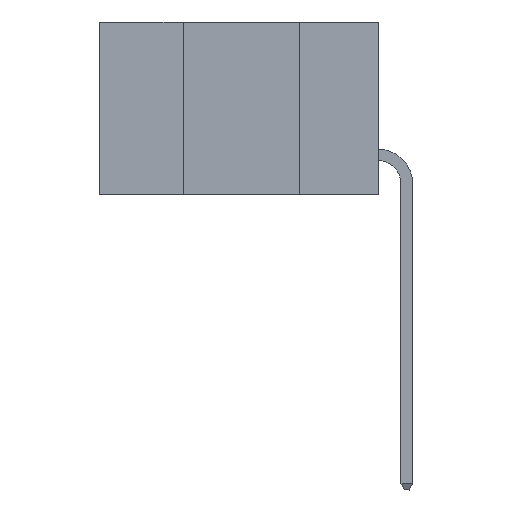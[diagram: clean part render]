
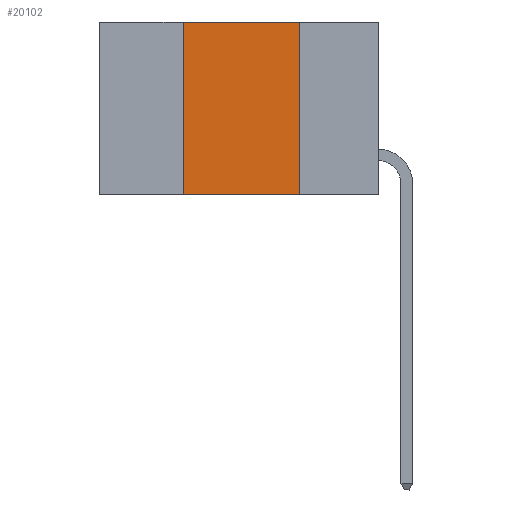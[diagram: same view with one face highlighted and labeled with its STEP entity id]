
A CAD part, left-side view. The second image highlights one B-rep face of the part: STEP entity #20102.
In plain terms, the highlighted planar face has unit normal (-1, 0, 0).
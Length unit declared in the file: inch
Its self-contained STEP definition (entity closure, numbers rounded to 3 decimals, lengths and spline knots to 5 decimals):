
#1355 = VECTOR ( 'NONE', #16091, 39.37008 ) ;
#1516 = EDGE_CURVE ( 'NONE', #18307, #8647, #14158, .T. ) ;
#3431 = PLANE ( 'NONE',  #28466 ) ;
#4315 = CARTESIAN_POINT ( 'NONE',  ( 0., 0.42, 0. ) ) ;
#7027 = LINE ( 'NONE', #16688, #25282 ) ;
#8188 = LINE ( 'NONE', #4315, #19424 ) ;
#8274 = DIRECTION ( 'NONE',  ( 1., 0., 0. ) ) ;
#8341 = CARTESIAN_POINT ( 'NONE',  ( 0., 0.17, 0. ) ) ;
#8647 = VERTEX_POINT ( 'NONE', #8341 ) ;
#9548 = DIRECTION ( 'NONE',  ( 0., -1., 0. ) ) ;
#10759 = ORIENTED_EDGE ( 'NONE', *, *, #26162, .F. ) ;
#11028 = VERTEX_POINT ( 'NONE', #11804 ) ;
#11540 = ORIENTED_EDGE ( 'NONE', *, *, #26784, .F. ) ;
#11804 = CARTESIAN_POINT ( 'NONE',  ( 0., 0.17, -0.37 ) ) ;
#13955 = EDGE_LOOP ( 'NONE', ( #10759, #23388, #11540, #28905 ) ) ;
#14158 = LINE ( 'NONE', #28954, #1355 ) ;
#16091 = DIRECTION ( 'NONE',  ( 0., -1., 0. ) ) ;
#16284 = VERTEX_POINT ( 'NONE', #22019 ) ;
#16291 = DIRECTION ( 'NONE',  ( 0., 0., 1. ) ) ;
#16688 = CARTESIAN_POINT ( 'NONE',  ( 0., 0.6, -0.37 ) ) ;
#18307 = VERTEX_POINT ( 'NONE', #29461 ) ;
#18661 = FACE_OUTER_BOUND ( 'NONE', #13955, .T. ) ;
#18730 = CARTESIAN_POINT ( 'NONE',  ( 0., 0.17, 0. ) ) ;
#19424 = VECTOR ( 'NONE', #16291, 39.37008 ) ;
#20102 = ADVANCED_FACE ( 'NONE', ( #18661 ), #3431, .F. ) ;
#22019 = CARTESIAN_POINT ( 'NONE',  ( 0., 0.42, -0.37 ) ) ;
#23388 = ORIENTED_EDGE ( 'NONE', *, *, #1516, .F. ) ;
#24928 = DIRECTION ( 'NONE',  ( 0., 0., -1. ) ) ;
#25282 = VECTOR ( 'NONE', #9548, 39.37008 ) ;
#25345 = VECTOR ( 'NONE', #28113, 39.37008 ) ;
#26162 = EDGE_CURVE ( 'NONE', #8647, #11028, #26773, .T. ) ;
#26773 = LINE ( 'NONE', #18730, #25345 ) ;
#26784 = EDGE_CURVE ( 'NONE', #16284, #18307, #8188, .T. ) ;
#27134 = CARTESIAN_POINT ( 'NONE',  ( 0., 0.6, 0. ) ) ;
#28113 = DIRECTION ( 'NONE',  ( 0., 0., -1. ) ) ;
#28466 = AXIS2_PLACEMENT_3D ( 'NONE', #27134, #8274, #24928 ) ;
#28905 = ORIENTED_EDGE ( 'NONE', *, *, #28980, .T. ) ;
#28954 = CARTESIAN_POINT ( 'NONE',  ( 0., 0.6, 0. ) ) ;
#28980 = EDGE_CURVE ( 'NONE', #16284, #11028, #7027, .T. ) ;
#29461 = CARTESIAN_POINT ( 'NONE',  ( 0., 0.42, 0. ) ) ;
